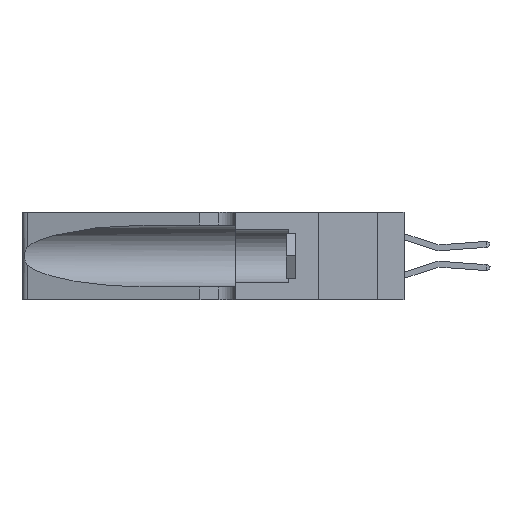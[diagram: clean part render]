
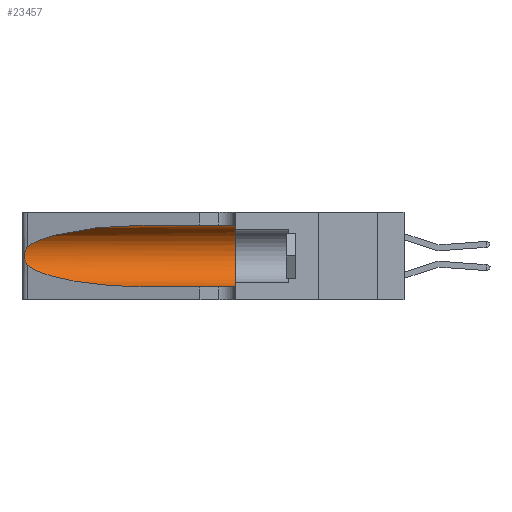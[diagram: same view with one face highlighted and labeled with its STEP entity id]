
A CAD part, left-side view. The second image highlights one B-rep face of the part: STEP entity #23457.
In plain terms, the highlighted cylindrical face has radius 3.308 mm (diameter 6.617 mm), a partial arc.
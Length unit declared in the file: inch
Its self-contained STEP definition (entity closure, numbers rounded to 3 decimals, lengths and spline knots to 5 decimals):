
#444 = CARTESIAN_POINT ( 'NONE',  ( 0.25555, 1.22993, 0.14849 ) ) ;
#1124 = CARTESIAN_POINT ( 'NONE',  ( 0.25487, 1.22718, 0.22369 ) ) ;
#1226 = VERTEX_POINT ( 'NONE', #18176 ) ;
#2825 = CARTESIAN_POINT ( 'NONE',  ( 0.18966, 0.96281, 0.05475 ) ) ;
#4656 = LINE ( 'NONE', #45641, #13000 ) ;
#6210 = CARTESIAN_POINT ( 'NONE',  ( 0.25487, 1.22718, 0.14631 ) ) ;
#6690 =( BOUNDED_CURVE ( )  B_SPLINE_CURVE ( 3, ( #10833, #39004, #7424, #32061 ),
 .UNSPECIFIED., .F., .F. ) 
 B_SPLINE_CURVE_WITH_KNOTS ( ( 4, 4 ),
 ( 1.5708, 2.84003 ),
 .UNSPECIFIED. ) 
 CURVE ( )  GEOMETRIC_REPRESENTATION_ITEM ( )  RATIONAL_B_SPLINE_CURVE ( ( 1., 0.87, 0.87, 1. ) ) 
 REPRESENTATION_ITEM ( '' )  );
#7424 = CARTESIAN_POINT ( 'NONE',  ( 0.2373, 1.15595, 0.28018 ) ) ;
#7481 = CARTESIAN_POINT ( 'NONE',  ( 0.25787, 1.23484, 0.2124 ) ) ;
#10833 = CARTESIAN_POINT ( 'NONE',  ( 0.1305, 0.72297, 0.31525 ) ) ;
#11047 = CARTESIAN_POINT ( 'NONE',  ( 0.26018, 1.23835, 0.19895 ) ) ;
#12825 = CARTESIAN_POINT ( 'NONE',  ( 0.1305, 0.35, 0.185 ) ) ;
#13000 = VECTOR ( 'NONE', #42102, 39.37008 ) ;
#14251 = CARTESIAN_POINT ( 'NONE',  ( 0.1305, 1.61858, 0.05475 ) ) ;
#14609 = CARTESIAN_POINT ( 'NONE',  ( 0.26075, 1.23896, 0.178 ) ) ;
#14857 = VERTEX_POINT ( 'NONE', #22991 ) ;
#14940 = B_SPLINE_CURVE_WITH_KNOTS ( 'NONE', 3,
 ( #25107, #21576, #28647, #7481, #32115, #11047, #35691, #14609, #39206, #18192, #42758, #21733, #444, #25254 ),
 .UNSPECIFIED., .F., .F.,
 ( 4, 2, 2, 2, 2, 2, 4 ),
 ( 0., 0.00027, 0.00053, 0.00107, 0.0016, 0.00187, 0.00214 ),
 .UNSPECIFIED. ) ;
#15015 = AXIS2_PLACEMENT_3D ( 'NONE', #12825, #37451, #16387 ) ;
#16387 = DIRECTION ( 'NONE',  ( 0., 0., 1. ) ) ;
#16590 = EDGE_CURVE ( 'NONE', #38138, #14857, #4656, .T. ) ;
#17329 = FACE_OUTER_BOUND ( 'NONE', #34951, .T. ) ;
#18176 = CARTESIAN_POINT ( 'NONE',  ( 0.25487, 1.22718, 0.14631 ) ) ;
#18192 = CARTESIAN_POINT ( 'NONE',  ( 0.25856, 1.23593, 0.16098 ) ) ;
#18697 = CARTESIAN_POINT ( 'NONE',  ( 0.1305, 0.72297, 0.31525 ) ) ;
#19239 = ORIENTED_EDGE ( 'NONE', *, *, #27181, .T. ) ;
#19827 = CARTESIAN_POINT ( 'NONE',  ( 0.1305, 0.35, 0.05475 ) ) ;
#20502 = CARTESIAN_POINT ( 'NONE',  ( 0.2373, 1.15595, 0.08982 ) ) ;
#20887 = VERTEX_POINT ( 'NONE', #19827 ) ;
#21576 = CARTESIAN_POINT ( 'NONE',  ( 0.25555, 1.22994, 0.2215 ) ) ;
#21733 = CARTESIAN_POINT ( 'NONE',  ( 0.25639, 1.23186, 0.15144 ) ) ;
#22991 = CARTESIAN_POINT ( 'NONE',  ( 0.1305, 0.35, 0.31525 ) ) ;
#23457 = ADVANCED_FACE ( 'NONE', ( #17329 ), #44267, .F. ) ;
#23504 = CIRCLE ( 'NONE', #15015, 0.13025 ) ;
#25107 = CARTESIAN_POINT ( 'NONE',  ( 0.25487, 1.22718, 0.22369 ) ) ;
#25254 = CARTESIAN_POINT ( 'NONE',  ( 0.25487, 1.22718, 0.14631 ) ) ;
#26879 = ORIENTED_EDGE ( 'NONE', *, *, #16590, .F. ) ;
#27181 = EDGE_CURVE ( 'NONE', #1226, #30988, #31275, .T. ) ;
#27574 = CARTESIAN_POINT ( 'NONE',  ( 0.1305, 0.72297, 0.05475 ) ) ;
#28082 = AXIS2_PLACEMENT_3D ( 'NONE', #32190, #39284, #35778 ) ;
#28647 = CARTESIAN_POINT ( 'NONE',  ( 0.25639, 1.23184, 0.21858 ) ) ;
#30988 = VERTEX_POINT ( 'NONE', #36722 ) ;
#31211 = ORIENTED_EDGE ( 'NONE', *, *, #31223, .F. ) ;
#31223 = EDGE_CURVE ( 'NONE', #14857, #20887, #23504, .T. ) ;
#31275 =( BOUNDED_CURVE ( )  B_SPLINE_CURVE ( 3, ( #6210, #20502, #2825, #27574 ),
 .UNSPECIFIED., .F., .T. ) 
 B_SPLINE_CURVE_WITH_KNOTS ( ( 4, 4 ),
 ( 3.44316, 4.71239 ),
 .UNSPECIFIED. ) 
 CURVE ( )  GEOMETRIC_REPRESENTATION_ITEM ( )  RATIONAL_B_SPLINE_CURVE ( ( 1., 0.87, 0.87, 1. ) ) 
 REPRESENTATION_ITEM ( '' )  );
#32061 = CARTESIAN_POINT ( 'NONE',  ( 0.25487, 1.22718, 0.22369 ) ) ;
#32115 = CARTESIAN_POINT ( 'NONE',  ( 0.25854, 1.2359, 0.20912 ) ) ;
#32190 = CARTESIAN_POINT ( 'NONE',  ( 0.1305, 1.61858, 0.185 ) ) ;
#33060 = EDGE_CURVE ( 'NONE', #30988, #20887, #34546, .T. ) ;
#34546 = LINE ( 'NONE', #14251, #41698 ) ;
#34951 = EDGE_LOOP ( 'NONE', ( #35649, #35201, #19239, #44487, #31211, #26879 ) ) ;
#35201 = ORIENTED_EDGE ( 'NONE', *, *, #35434, .T. ) ;
#35434 = EDGE_CURVE ( 'NONE', #38171, #1226, #14940, .T. ) ;
#35649 = ORIENTED_EDGE ( 'NONE', *, *, #36022, .T. ) ;
#35691 = CARTESIAN_POINT ( 'NONE',  ( 0.26075, 1.23896, 0.19203 ) ) ;
#35778 = DIRECTION ( 'NONE',  ( 0., 0., -1. ) ) ;
#36022 = EDGE_CURVE ( 'NONE', #38138, #38171, #6690, .T. ) ;
#36722 = CARTESIAN_POINT ( 'NONE',  ( 0.1305, 0.72297, 0.05475 ) ) ;
#37451 = DIRECTION ( 'NONE',  ( 0., 1., 0. ) ) ;
#38138 = VERTEX_POINT ( 'NONE', #18697 ) ;
#38171 = VERTEX_POINT ( 'NONE', #1124 ) ;
#39004 = CARTESIAN_POINT ( 'NONE',  ( 0.18966, 0.96281, 0.31525 ) ) ;
#39206 = CARTESIAN_POINT ( 'NONE',  ( 0.26017, 1.23833, 0.17102 ) ) ;
#39284 = DIRECTION ( 'NONE',  ( 0., -1., 0. ) ) ;
#41698 = VECTOR ( 'NONE', #42426, 39.37008 ) ;
#42102 = DIRECTION ( 'NONE',  ( 0., -1., 0. ) ) ;
#42426 = DIRECTION ( 'NONE',  ( 0., -1., 0. ) ) ;
#42758 = CARTESIAN_POINT ( 'NONE',  ( 0.25789, 1.23486, 0.15765 ) ) ;
#44267 = CYLINDRICAL_SURFACE ( 'NONE', #28082, 0.13025 ) ;
#44487 = ORIENTED_EDGE ( 'NONE', *, *, #33060, .T. ) ;
#45641 = CARTESIAN_POINT ( 'NONE',  ( 0.1305, 1.61858, 0.31525 ) ) ;
